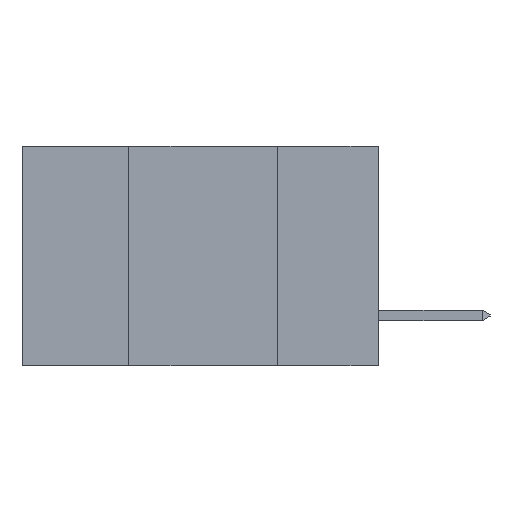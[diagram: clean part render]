
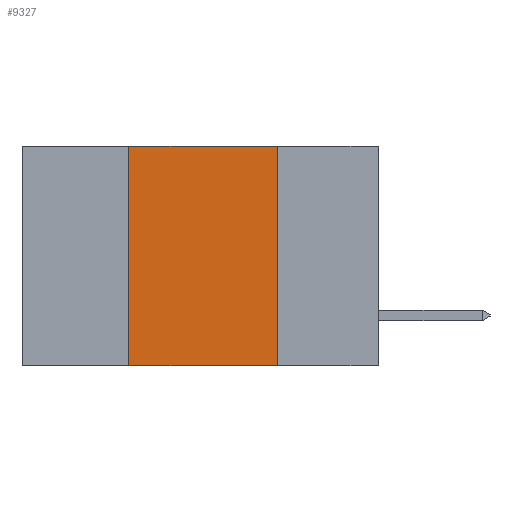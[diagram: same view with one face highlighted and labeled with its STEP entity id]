
A CAD part, left-side view. The second image highlights one B-rep face of the part: STEP entity #9327.
In plain terms, the highlighted planar face has unit normal (-1, 0, 0).
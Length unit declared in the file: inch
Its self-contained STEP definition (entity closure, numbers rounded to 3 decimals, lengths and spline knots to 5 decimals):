
#973 = CARTESIAN_POINT ( 'NONE',  ( 0., 0.6, 0. ) ) ;
#2217 = DIRECTION ( 'NONE',  ( 0., -1., 0. ) ) ;
#2647 = LINE ( 'NONE', #15830, #14979 ) ;
#2752 = EDGE_CURVE ( 'NONE', #5483, #9607, #15534, .T. ) ;
#2893 = FACE_OUTER_BOUND ( 'NONE', #9016, .T. ) ;
#2961 = EDGE_CURVE ( 'NONE', #9607, #13852, #14618, .T. ) ;
#4035 = ORIENTED_EDGE ( 'NONE', *, *, #2961, .F. ) ;
#5483 = VERTEX_POINT ( 'NONE', #18237 ) ;
#7030 = EDGE_CURVE ( 'NONE', #5483, #10979, #2647, .T. ) ;
#7526 = VECTOR ( 'NONE', #13372, 39.37008 ) ;
#9016 = EDGE_LOOP ( 'NONE', ( #9166, #4035, #18561, #11286 ) ) ;
#9166 = ORIENTED_EDGE ( 'NONE', *, *, #10902, .F. ) ;
#9327 = ADVANCED_FACE ( 'NONE', ( #2893 ), #17152, .F. ) ;
#9607 = VERTEX_POINT ( 'NONE', #11949 ) ;
#9938 = AXIS2_PLACEMENT_3D ( 'NONE', #18319, #18343, #19802 ) ;
#10902 = EDGE_CURVE ( 'NONE', #13852, #10979, #13890, .T. ) ;
#10979 = VERTEX_POINT ( 'NONE', #16049 ) ;
#11045 = DIRECTION ( 'NONE',  ( 0., 0., -1. ) ) ;
#11286 = ORIENTED_EDGE ( 'NONE', *, *, #7030, .T. ) ;
#11435 = CARTESIAN_POINT ( 'NONE',  ( 0., 0.17, 0. ) ) ;
#11949 = CARTESIAN_POINT ( 'NONE',  ( 0., 0.42, 0. ) ) ;
#13372 = DIRECTION ( 'NONE',  ( 0., 0., 1. ) ) ;
#13852 = VERTEX_POINT ( 'NONE', #11435 ) ;
#13890 = LINE ( 'NONE', #18958, #17627 ) ;
#14618 = LINE ( 'NONE', #973, #18318 ) ;
#14979 = VECTOR ( 'NONE', #15572, 39.37008 ) ;
#15217 = CARTESIAN_POINT ( 'NONE',  ( 0., 0.42, -0.37 ) ) ;
#15534 = LINE ( 'NONE', #15217, #7526 ) ;
#15572 = DIRECTION ( 'NONE',  ( 0., -1., 0. ) ) ;
#15830 = CARTESIAN_POINT ( 'NONE',  ( 0., 0.6, -0.37 ) ) ;
#16049 = CARTESIAN_POINT ( 'NONE',  ( 0., 0.17, -0.37 ) ) ;
#17152 = PLANE ( 'NONE',  #9938 ) ;
#17627 = VECTOR ( 'NONE', #11045, 39.37008 ) ;
#18237 = CARTESIAN_POINT ( 'NONE',  ( 0., 0.42, -0.37 ) ) ;
#18318 = VECTOR ( 'NONE', #2217, 39.37008 ) ;
#18319 = CARTESIAN_POINT ( 'NONE',  ( 0., 0.6, 0. ) ) ;
#18343 = DIRECTION ( 'NONE',  ( 1., 0., 0. ) ) ;
#18561 = ORIENTED_EDGE ( 'NONE', *, *, #2752, .F. ) ;
#18958 = CARTESIAN_POINT ( 'NONE',  ( 0., 0.17, -0.37 ) ) ;
#19802 = DIRECTION ( 'NONE',  ( 0., 0., -1. ) ) ;
